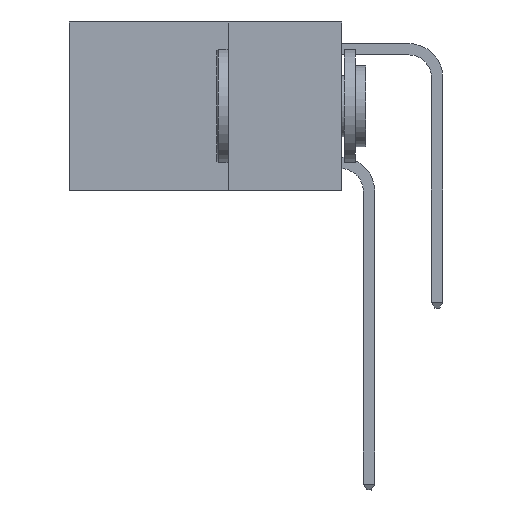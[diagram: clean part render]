
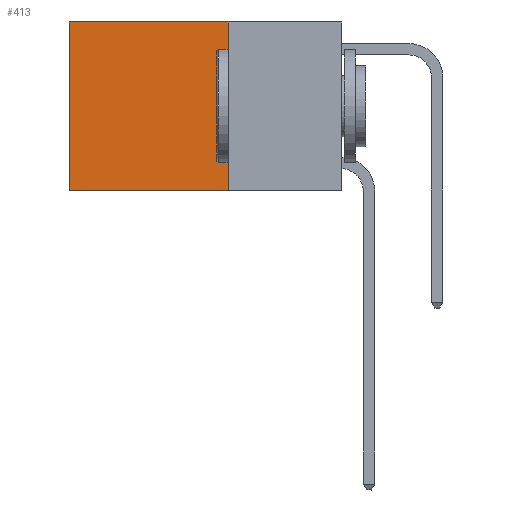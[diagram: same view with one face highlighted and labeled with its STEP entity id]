
A CAD part, left-side view. The second image highlights one B-rep face of the part: STEP entity #413.
In plain terms, the highlighted planar face has unit normal (-1, 0, 0).
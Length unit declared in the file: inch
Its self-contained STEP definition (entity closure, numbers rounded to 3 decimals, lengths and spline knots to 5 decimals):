
#117 = CARTESIAN_POINT ( 'NONE',  ( 0.2625, 0.25, 0. ) ) ;
#167 = CARTESIAN_POINT ( 'NONE',  ( 0.2625, 0.25, -0.37 ) ) ;
#413 = ADVANCED_FACE ( 'NONE', ( #9922 ), #14909, .F. ) ;
#1593 = VECTOR ( 'NONE', #12021, 39.37008 ) ;
#2119 = VERTEX_POINT ( 'NONE', #6404 ) ;
#2742 = EDGE_CURVE ( 'NONE', #6901, #14572, #5303, .T. ) ;
#3203 = CARTESIAN_POINT ( 'NONE',  ( 0.2625, 0.25, -0.37 ) ) ;
#3205 = DIRECTION ( 'NONE',  ( 0., 0., -1. ) ) ;
#3601 = CARTESIAN_POINT ( 'NONE',  ( 0.2625, 0.25, 0. ) ) ;
#3771 = CARTESIAN_POINT ( 'NONE',  ( 0.2625, 0.25, 0. ) ) ;
#4099 = AXIS2_PLACEMENT_3D ( 'NONE', #3601, #8072, #7916 ) ;
#4523 = CARTESIAN_POINT ( 'NONE',  ( 0.2625, 0.6, 0. ) ) ;
#4571 = EDGE_CURVE ( 'NONE', #14572, #2119, #15675, .T. ) ;
#5303 = LINE ( 'NONE', #117, #14867 ) ;
#5316 = EDGE_CURVE ( 'NONE', #8270, #2119, #11976, .T. ) ;
#5701 = DIRECTION ( 'NONE',  ( 0., 1., 0. ) ) ;
#6404 = CARTESIAN_POINT ( 'NONE',  ( 0.2625, 0.6, -0.37 ) ) ;
#6901 = VERTEX_POINT ( 'NONE', #3771 ) ;
#7572 = ORIENTED_EDGE ( 'NONE', *, *, #7705, .F. ) ;
#7705 = EDGE_CURVE ( 'NONE', #6901, #8270, #10868, .T. ) ;
#7916 = DIRECTION ( 'NONE',  ( 0., 0., -1. ) ) ;
#8072 = DIRECTION ( 'NONE',  ( 1., 0., 0. ) ) ;
#8270 = VERTEX_POINT ( 'NONE', #167 ) ;
#9278 = DIRECTION ( 'NONE',  ( 0., 1., 0. ) ) ;
#9345 = ORIENTED_EDGE ( 'NONE', *, *, #5316, .F. ) ;
#9922 = FACE_OUTER_BOUND ( 'NONE', #16174, .T. ) ;
#10094 = VECTOR ( 'NONE', #3205, 39.37008 ) ;
#10868 = LINE ( 'NONE', #15887, #1593 ) ;
#11976 = LINE ( 'NONE', #3203, #12742 ) ;
#12021 = DIRECTION ( 'NONE',  ( 0., 0., -1. ) ) ;
#12742 = VECTOR ( 'NONE', #5701, 39.37008 ) ;
#12780 = ORIENTED_EDGE ( 'NONE', *, *, #2742, .T. ) ;
#13127 = ORIENTED_EDGE ( 'NONE', *, *, #4571, .T. ) ;
#14572 = VERTEX_POINT ( 'NONE', #16129 ) ;
#14867 = VECTOR ( 'NONE', #9278, 39.37008 ) ;
#14909 = PLANE ( 'NONE',  #4099 ) ;
#15675 = LINE ( 'NONE', #4523, #10094 ) ;
#15887 = CARTESIAN_POINT ( 'NONE',  ( 0.2625, 0.25, 0. ) ) ;
#16129 = CARTESIAN_POINT ( 'NONE',  ( 0.2625, 0.6, 0. ) ) ;
#16174 = EDGE_LOOP ( 'NONE', ( #13127, #9345, #7572, #12780 ) ) ;
